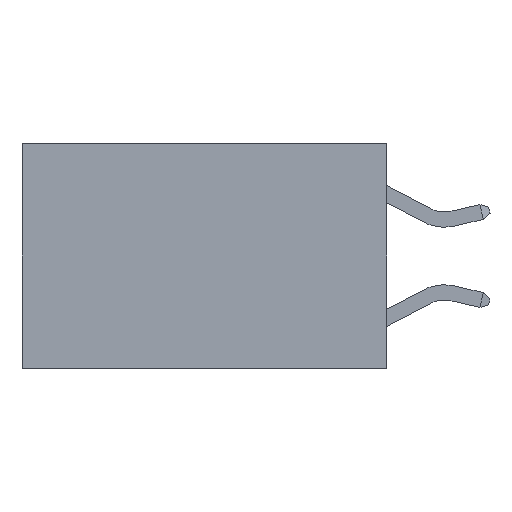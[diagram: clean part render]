
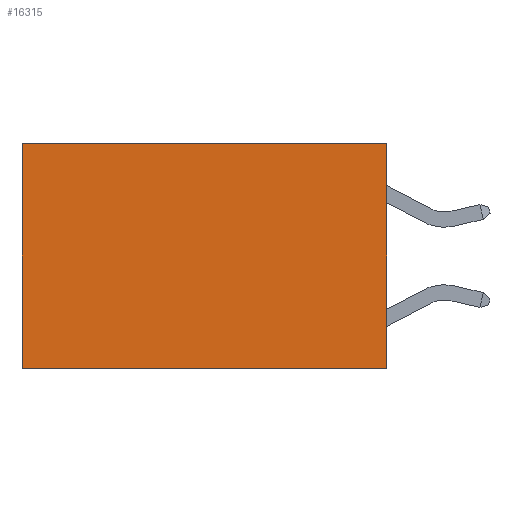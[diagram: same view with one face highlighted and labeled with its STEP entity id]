
A CAD part, left-side view. The second image highlights one B-rep face of the part: STEP entity #16315.
In plain terms, the highlighted planar face has unit normal (-1, 0, 0).
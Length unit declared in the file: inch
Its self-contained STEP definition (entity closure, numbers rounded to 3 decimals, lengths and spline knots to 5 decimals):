
#640 = VECTOR ( 'NONE', #26918, 39.37008 ) ;
#1219 = CARTESIAN_POINT ( 'NONE',  ( 0.2625, 0., 0. ) ) ;
#1337 = DIRECTION ( 'NONE',  ( 1., 0., 0. ) ) ;
#3907 = VERTEX_POINT ( 'NONE', #12623 ) ;
#5287 = EDGE_LOOP ( 'NONE', ( #22336, #12028, #14969, #9069 ) ) ;
#5515 = EDGE_CURVE ( 'NONE', #22423, #3907, #20867, .T. ) ;
#5608 = CARTESIAN_POINT ( 'NONE',  ( 0.2625, 0., -0.37 ) ) ;
#5673 = CARTESIAN_POINT ( 'NONE',  ( 0.2625, 0., 0. ) ) ;
#7672 = LINE ( 'NONE', #5608, #12878 ) ;
#7851 = DIRECTION ( 'NONE',  ( 0., 1., 0. ) ) ;
#8521 = DIRECTION ( 'NONE',  ( 0., 0., -1. ) ) ;
#9069 = ORIENTED_EDGE ( 'NONE', *, *, #5515, .T. ) ;
#9209 = VECTOR ( 'NONE', #26775, 39.37008 ) ;
#9229 = EDGE_CURVE ( 'NONE', #3907, #23306, #18240, .T. ) ;
#11600 = EDGE_CURVE ( 'NONE', #22423, #27131, #28005, .T. ) ;
#12028 = ORIENTED_EDGE ( 'NONE', *, *, #23649, .F. ) ;
#12360 = PLANE ( 'NONE',  #14155 ) ;
#12623 = CARTESIAN_POINT ( 'NONE',  ( 0.2625, 0.6, 0. ) ) ;
#12878 = VECTOR ( 'NONE', #7851, 39.37008 ) ;
#14155 = AXIS2_PLACEMENT_3D ( 'NONE', #5673, #1337, #16753 ) ;
#14969 = ORIENTED_EDGE ( 'NONE', *, *, #11600, .F. ) ;
#15477 = CARTESIAN_POINT ( 'NONE',  ( 0.2625, 0.6, -0.37 ) ) ;
#16315 = ADVANCED_FACE ( 'NONE', ( #21849 ), #12360, .F. ) ;
#16753 = DIRECTION ( 'NONE',  ( 0., 0., -1. ) ) ;
#18240 = LINE ( 'NONE', #24740, #640 ) ;
#20867 = LINE ( 'NONE', #22473, #9209 ) ;
#21849 = FACE_OUTER_BOUND ( 'NONE', #5287, .T. ) ;
#22154 = CARTESIAN_POINT ( 'NONE',  ( 0.2625, 0., -0.37 ) ) ;
#22336 = ORIENTED_EDGE ( 'NONE', *, *, #9229, .T. ) ;
#22423 = VERTEX_POINT ( 'NONE', #1219 ) ;
#22473 = CARTESIAN_POINT ( 'NONE',  ( 0.2625, 0., 0. ) ) ;
#23306 = VERTEX_POINT ( 'NONE', #15477 ) ;
#23649 = EDGE_CURVE ( 'NONE', #27131, #23306, #7672, .T. ) ;
#24740 = CARTESIAN_POINT ( 'NONE',  ( 0.2625, 0.6, 0. ) ) ;
#26036 = CARTESIAN_POINT ( 'NONE',  ( 0.2625, 0., 0. ) ) ;
#26775 = DIRECTION ( 'NONE',  ( 0., 1., 0. ) ) ;
#26918 = DIRECTION ( 'NONE',  ( 0., 0., -1. ) ) ;
#27131 = VERTEX_POINT ( 'NONE', #22154 ) ;
#27328 = VECTOR ( 'NONE', #8521, 39.37008 ) ;
#28005 = LINE ( 'NONE', #26036, #27328 ) ;
